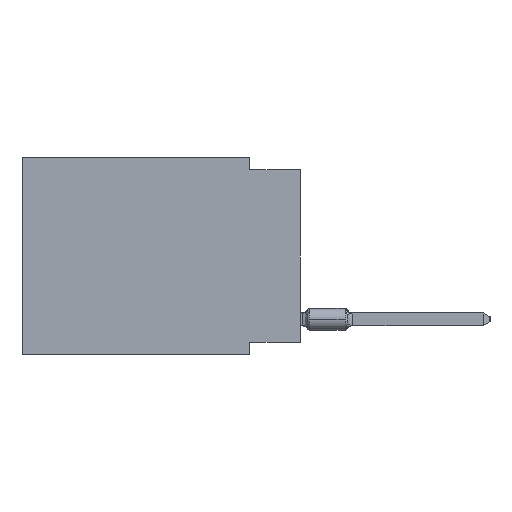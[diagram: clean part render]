
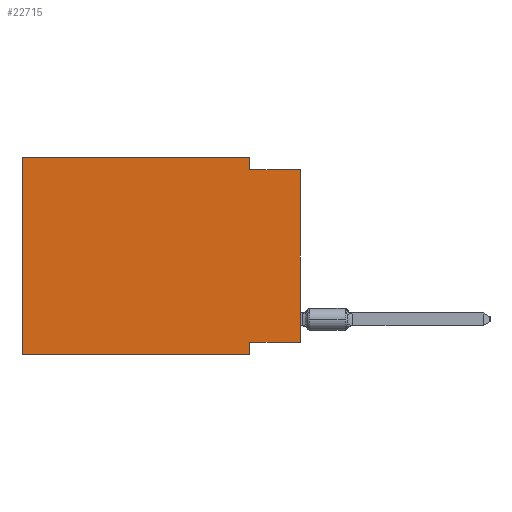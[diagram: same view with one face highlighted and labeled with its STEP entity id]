
A CAD part, left-side view. The second image highlights one B-rep face of the part: STEP entity #22715.
In plain terms, the highlighted planar face has unit normal (-1, 0, 0).
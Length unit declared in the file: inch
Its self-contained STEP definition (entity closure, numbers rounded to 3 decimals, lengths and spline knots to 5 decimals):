
#739 = LINE ( 'NONE', #2181, #9622 ) ;
#1951 = LINE ( 'NONE', #30388, #35903 ) ;
#2039 = DIRECTION ( 'NONE',  ( 0., 0., -1. ) ) ;
#2047 = VECTOR ( 'NONE', #25617, 39.37008 ) ;
#2181 = CARTESIAN_POINT ( 'NONE',  ( 0., 0.55, 0. ) ) ;
#4226 = EDGE_CURVE ( 'NONE', #14824, #12524, #20775, .T. ) ;
#4876 = DIRECTION ( 'NONE',  ( 0., 1., 0. ) ) ;
#6606 = CARTESIAN_POINT ( 'NONE',  ( 0., 0.55, 0. ) ) ;
#7423 = LINE ( 'NONE', #8517, #16074 ) ;
#8517 = CARTESIAN_POINT ( 'NONE',  ( 0., 0.55, -0.39 ) ) ;
#8676 = EDGE_LOOP ( 'NONE', ( #50995, #38436, #57264, #37055, #30345, #39972, #26965, #68706 ) ) ;
#9622 = VECTOR ( 'NONE', #13637, 39.37008 ) ;
#9711 = DIRECTION ( 'NONE',  ( 0., -1., 0. ) ) ;
#11176 = VERTEX_POINT ( 'NONE', #52603 ) ;
#12180 = CARTESIAN_POINT ( 'NONE',  ( 0., 0.1, -0.025 ) ) ;
#12524 = VERTEX_POINT ( 'NONE', #18678 ) ;
#13637 = DIRECTION ( 'NONE',  ( 0., -1., 0. ) ) ;
#14824 = VERTEX_POINT ( 'NONE', #12180 ) ;
#15256 = LINE ( 'NONE', #26715, #2047 ) ;
#16074 = VECTOR ( 'NONE', #48055, 39.37008 ) ;
#16255 = AXIS2_PLACEMENT_3D ( 'NONE', #69686, #52352, #63813 ) ;
#17244 = CARTESIAN_POINT ( 'NONE',  ( 0., 0.55, 0. ) ) ;
#17422 = EDGE_CURVE ( 'NONE', #56492, #59826, #7423, .T. ) ;
#18678 = CARTESIAN_POINT ( 'NONE',  ( 0., 0., -0.025 ) ) ;
#20392 = EDGE_CURVE ( 'NONE', #11176, #40073, #71030, .T. ) ;
#20775 = LINE ( 'NONE', #21868, #68304 ) ;
#20995 = EDGE_CURVE ( 'NONE', #56492, #59246, #56175, .T. ) ;
#21868 = CARTESIAN_POINT ( 'NONE',  ( 0., 0., -0.025 ) ) ;
#22715 = ADVANCED_FACE ( 'NONE', ( #25343 ), #24242, .F. ) ;
#24242 = PLANE ( 'NONE',  #16255 ) ;
#25343 = FACE_OUTER_BOUND ( 'NONE', #8676, .T. ) ;
#25617 = DIRECTION ( 'NONE',  ( 0., 0., 1. ) ) ;
#26715 = CARTESIAN_POINT ( 'NONE',  ( 0., 0., 0. ) ) ;
#26965 = ORIENTED_EDGE ( 'NONE', *, *, #32688, .F. ) ;
#27745 = CARTESIAN_POINT ( 'NONE',  ( 0., 0.55, -0.39 ) ) ;
#28682 = CARTESIAN_POINT ( 'NONE',  ( 0., 0.1, 0. ) ) ;
#30345 = ORIENTED_EDGE ( 'NONE', *, *, #20995, .F. ) ;
#30388 = CARTESIAN_POINT ( 'NONE',  ( 0., 0.1, -0.39 ) ) ;
#32206 = VERTEX_POINT ( 'NONE', #73025 ) ;
#32688 = EDGE_CURVE ( 'NONE', #40073, #59826, #1951, .T. ) ;
#35189 = CARTESIAN_POINT ( 'NONE',  ( 0., 0.1, -0.365 ) ) ;
#35418 = VECTOR ( 'NONE', #2039, 39.37008 ) ;
#35903 = VECTOR ( 'NONE', #64056, 39.37008 ) ;
#37055 = ORIENTED_EDGE ( 'NONE', *, *, #61718, .F. ) ;
#37472 = EDGE_CURVE ( 'NONE', #32206, #14824, #69284, .T. ) ;
#38436 = ORIENTED_EDGE ( 'NONE', *, *, #4226, .F. ) ;
#39972 = ORIENTED_EDGE ( 'NONE', *, *, #17422, .T. ) ;
#40073 = VERTEX_POINT ( 'NONE', #35189 ) ;
#44600 = VECTOR ( 'NONE', #50618, 39.37008 ) ;
#48055 = DIRECTION ( 'NONE',  ( 0., -1., 0. ) ) ;
#50600 = VECTOR ( 'NONE', #4876, 39.37008 ) ;
#50618 = DIRECTION ( 'NONE',  ( 0., 0., 1. ) ) ;
#50995 = ORIENTED_EDGE ( 'NONE', *, *, #54803, .T. ) ;
#52352 = DIRECTION ( 'NONE',  ( 1., 0., 0. ) ) ;
#52603 = CARTESIAN_POINT ( 'NONE',  ( 0., 0., -0.365 ) ) ;
#54803 = EDGE_CURVE ( 'NONE', #11176, #12524, #15256, .T. ) ;
#56175 = LINE ( 'NONE', #6606, #44600 ) ;
#56492 = VERTEX_POINT ( 'NONE', #27745 ) ;
#57264 = ORIENTED_EDGE ( 'NONE', *, *, #37472, .F. ) ;
#59246 = VERTEX_POINT ( 'NONE', #17244 ) ;
#59826 = VERTEX_POINT ( 'NONE', #69579 ) ;
#61718 = EDGE_CURVE ( 'NONE', #59246, #32206, #739, .T. ) ;
#63813 = DIRECTION ( 'NONE',  ( 0., 0., -1. ) ) ;
#64056 = DIRECTION ( 'NONE',  ( 0., 0., -1. ) ) ;
#67330 = CARTESIAN_POINT ( 'NONE',  ( 0., 0., -0.365 ) ) ;
#68304 = VECTOR ( 'NONE', #9711, 39.37008 ) ;
#68706 = ORIENTED_EDGE ( 'NONE', *, *, #20392, .F. ) ;
#69284 = LINE ( 'NONE', #28682, #35418 ) ;
#69579 = CARTESIAN_POINT ( 'NONE',  ( 0., 0.1, -0.39 ) ) ;
#69686 = CARTESIAN_POINT ( 'NONE',  ( 0., 0.55, 0. ) ) ;
#71030 = LINE ( 'NONE', #67330, #50600 ) ;
#73025 = CARTESIAN_POINT ( 'NONE',  ( 0., 0.1, 0. ) ) ;
